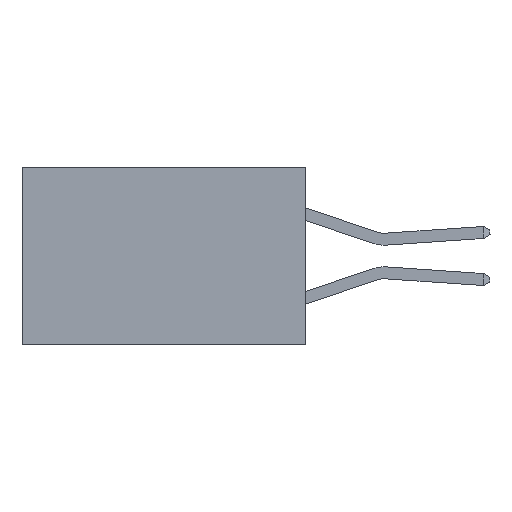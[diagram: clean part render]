
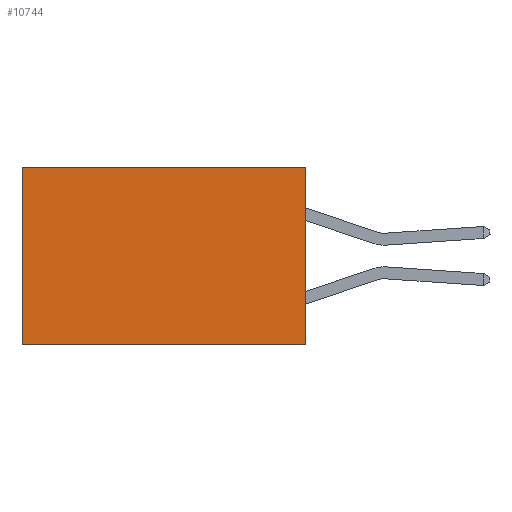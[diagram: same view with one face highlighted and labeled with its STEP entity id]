
A CAD part, left-side view. The second image highlights one B-rep face of the part: STEP entity #10744.
In plain terms, the highlighted planar face has unit normal (-1, 0, 0).
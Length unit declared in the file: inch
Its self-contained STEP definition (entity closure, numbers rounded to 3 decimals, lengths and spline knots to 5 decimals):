
#1960 = CARTESIAN_POINT ( 'NONE',  ( 0.277, 0., -0.37 ) ) ;
#3292 = LINE ( 'NONE', #24415, #28267 ) ;
#4155 = CARTESIAN_POINT ( 'NONE',  ( 0.277, 0., -0.37 ) ) ;
#4494 = FACE_OUTER_BOUND ( 'NONE', #15174, .T. ) ;
#5376 = LINE ( 'NONE', #19570, #11049 ) ;
#6349 = VERTEX_POINT ( 'NONE', #4155 ) ;
#8276 = DIRECTION ( 'NONE',  ( 1., 0., 0. ) ) ;
#9319 = ORIENTED_EDGE ( 'NONE', *, *, #24162, .F. ) ;
#10744 = ADVANCED_FACE ( 'NONE', ( #4494 ), #22771, .F. ) ;
#11049 = VECTOR ( 'NONE', #26720, 39.37008 ) ;
#11419 = VERTEX_POINT ( 'NONE', #15395 ) ;
#11521 = VERTEX_POINT ( 'NONE', #18193 ) ;
#14030 = VECTOR ( 'NONE', #28632, 39.37008 ) ;
#14648 = LINE ( 'NONE', #20173, #21115 ) ;
#14848 = DIRECTION ( 'NONE',  ( 0., 1., 0. ) ) ;
#15174 = EDGE_LOOP ( 'NONE', ( #18034, #9319, #30952, #25646 ) ) ;
#15395 = CARTESIAN_POINT ( 'NONE',  ( 0.277, 0.59, 0. ) ) ;
#15426 = CARTESIAN_POINT ( 'NONE',  ( 0.277, 0., -0.37 ) ) ;
#16039 = CARTESIAN_POINT ( 'NONE',  ( 0.277, 0., 0. ) ) ;
#17529 = VERTEX_POINT ( 'NONE', #16039 ) ;
#18034 = ORIENTED_EDGE ( 'NONE', *, *, #30529, .T. ) ;
#18193 = CARTESIAN_POINT ( 'NONE',  ( 0.277, 0.59, -0.37 ) ) ;
#19570 = CARTESIAN_POINT ( 'NONE',  ( 0.277, 0., 0. ) ) ;
#20173 = CARTESIAN_POINT ( 'NONE',  ( 0.277, 0.59, -0.37 ) ) ;
#21115 = VECTOR ( 'NONE', #22605, 39.37008 ) ;
#21488 = AXIS2_PLACEMENT_3D ( 'NONE', #15426, #8276, #25208 ) ;
#21651 = EDGE_CURVE ( 'NONE', #17529, #11419, #5376, .T. ) ;
#22605 = DIRECTION ( 'NONE',  ( 0., 0., -1. ) ) ;
#22771 = PLANE ( 'NONE',  #21488 ) ;
#22781 = LINE ( 'NONE', #1960, #14030 ) ;
#24162 = EDGE_CURVE ( 'NONE', #6349, #11521, #3292, .T. ) ;
#24415 = CARTESIAN_POINT ( 'NONE',  ( 0.277, 0., -0.37 ) ) ;
#25208 = DIRECTION ( 'NONE',  ( 0., 0., -1. ) ) ;
#25646 = ORIENTED_EDGE ( 'NONE', *, *, #21651, .T. ) ;
#26720 = DIRECTION ( 'NONE',  ( 0., 1., 0. ) ) ;
#28267 = VECTOR ( 'NONE', #14848, 39.37008 ) ;
#28312 = EDGE_CURVE ( 'NONE', #17529, #6349, #22781, .T. ) ;
#28632 = DIRECTION ( 'NONE',  ( 0., 0., -1. ) ) ;
#30529 = EDGE_CURVE ( 'NONE', #11419, #11521, #14648, .T. ) ;
#30952 = ORIENTED_EDGE ( 'NONE', *, *, #28312, .F. ) ;
